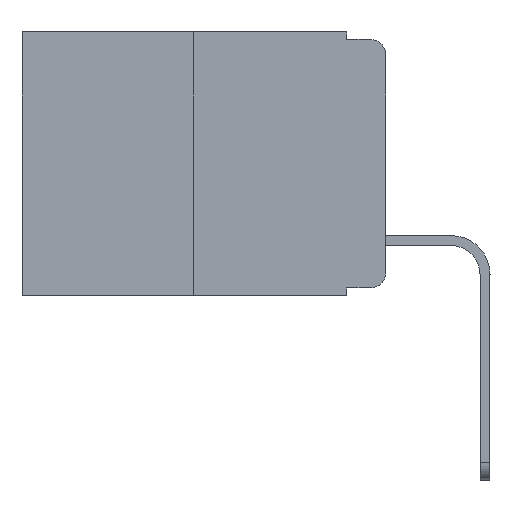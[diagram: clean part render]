
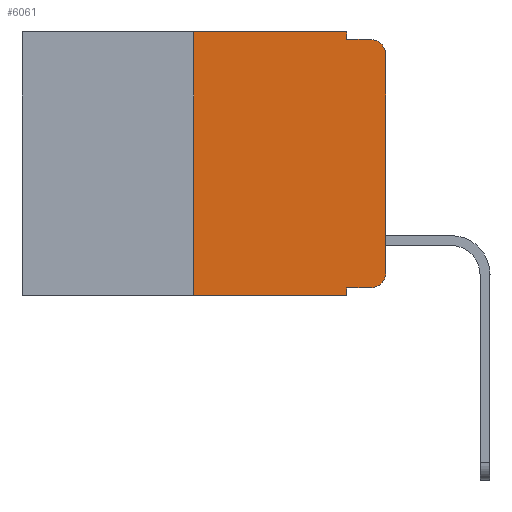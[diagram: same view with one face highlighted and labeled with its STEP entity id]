
A CAD part, left-side view. The second image highlights one B-rep face of the part: STEP entity #6061.
In plain terms, the highlighted planar face has unit normal (-1, 0, 0).
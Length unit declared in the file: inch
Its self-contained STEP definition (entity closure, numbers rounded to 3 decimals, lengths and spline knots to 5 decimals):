
#34 = VECTOR ( 'NONE', #3097, 39.37008 ) ;
#148 = CIRCLE ( 'NONE', #10623, 0.02 ) ;
#178 = ORIENTED_EDGE ( 'NONE', *, *, #2324, .T. ) ;
#459 = LINE ( 'NONE', #8525, #11110 ) ;
#597 = VERTEX_POINT ( 'NONE', #6587 ) ;
#667 = VERTEX_POINT ( 'NONE', #7694 ) ;
#918 = LINE ( 'NONE', #9375, #13182 ) ;
#1344 = EDGE_LOOP ( 'NONE', ( #1775, #178, #8103, #5149, #6812, #6428, #12021, #8382, #8187, #9135 ) ) ;
#1541 = CARTESIAN_POINT ( 'NONE',  ( 0., 0.02, -0.01 ) ) ;
#1775 = ORIENTED_EDGE ( 'NONE', *, *, #5289, .T. ) ;
#2139 = EDGE_CURVE ( 'NONE', #5920, #12277, #10236, .T. ) ;
#2301 = EDGE_CURVE ( 'NONE', #7351, #10772, #459, .T. ) ;
#2324 = EDGE_CURVE ( 'NONE', #7020, #2743, #148, .T. ) ;
#2660 = EDGE_CURVE ( 'NONE', #4343, #11978, #9646, .T. ) ;
#2743 = VERTEX_POINT ( 'NONE', #1541 ) ;
#2759 = CARTESIAN_POINT ( 'NONE',  ( 0., 0.473, 0. ) ) ;
#2847 = VECTOR ( 'NONE', #8816, 39.37008 ) ;
#2946 = DIRECTION ( 'NONE',  ( -1., 0., 0. ) ) ;
#2991 = CIRCLE ( 'NONE', #12866, 0.02 ) ;
#3029 = DIRECTION ( 'NONE',  ( 0., 0., -1. ) ) ;
#3097 = DIRECTION ( 'NONE',  ( 0., -1., 0. ) ) ;
#3358 = VECTOR ( 'NONE', #10687, 39.37008 ) ;
#3482 = LINE ( 'NONE', #8141, #8485 ) ;
#3493 = CARTESIAN_POINT ( 'NONE',  ( 0., 0.051, -0.333 ) ) ;
#3689 = LINE ( 'NONE', #3493, #3358 ) ;
#3695 = VECTOR ( 'NONE', #4351, 39.37008 ) ;
#3797 = DIRECTION ( 'NONE',  ( 0., 0., -1. ) ) ;
#4082 = CARTESIAN_POINT ( 'NONE',  ( 0., 0.051, -0.01 ) ) ;
#4132 = EDGE_CURVE ( 'NONE', #11978, #5920, #918, .T. ) ;
#4182 = CARTESIAN_POINT ( 'NONE',  ( 0., 0.051, -0.333 ) ) ;
#4343 = VERTEX_POINT ( 'NONE', #8898 ) ;
#4351 = DIRECTION ( 'NONE',  ( 0., 0., 1. ) ) ;
#4927 = DIRECTION ( 'NONE',  ( 0., 0., -1. ) ) ;
#5132 = CARTESIAN_POINT ( 'NONE',  ( 0., 0.25, 0. ) ) ;
#5149 = ORIENTED_EDGE ( 'NONE', *, *, #2139, .F. ) ;
#5204 = CARTESIAN_POINT ( 'NONE',  ( 0., 0.051, 0. ) ) ;
#5289 = EDGE_CURVE ( 'NONE', #667, #7020, #3482, .T. ) ;
#5399 = CARTESIAN_POINT ( 'NONE',  ( 0., 0.051, -0.01 ) ) ;
#5708 = FACE_OUTER_BOUND ( 'NONE', #1344, .T. ) ;
#5860 = CARTESIAN_POINT ( 'NONE',  ( 0., 0.25, 0. ) ) ;
#5920 = VERTEX_POINT ( 'NONE', #6330 ) ;
#6061 = ADVANCED_FACE ( 'NONE', ( #5708 ), #6921, .F. ) ;
#6109 = CARTESIAN_POINT ( 'NONE',  ( 0., 0.051, -0.343 ) ) ;
#6330 = CARTESIAN_POINT ( 'NONE',  ( 0., 0.051, 0. ) ) ;
#6428 = ORIENTED_EDGE ( 'NONE', *, *, #2660, .F. ) ;
#6587 = CARTESIAN_POINT ( 'NONE',  ( 0., 0.02, -0.333 ) ) ;
#6812 = ORIENTED_EDGE ( 'NONE', *, *, #4132, .F. ) ;
#6857 = EDGE_CURVE ( 'NONE', #12277, #2743, #13115, .T. ) ;
#6921 = PLANE ( 'NONE',  #10375 ) ;
#7020 = VERTEX_POINT ( 'NONE', #7466 ) ;
#7351 = VERTEX_POINT ( 'NONE', #4182 ) ;
#7466 = CARTESIAN_POINT ( 'NONE',  ( 0., 0., -0.03 ) ) ;
#7655 = CARTESIAN_POINT ( 'NONE',  ( 0., 0.473, -0.343 ) ) ;
#7694 = CARTESIAN_POINT ( 'NONE',  ( 0., 0., -0.313 ) ) ;
#8103 = ORIENTED_EDGE ( 'NONE', *, *, #6857, .F. ) ;
#8141 = CARTESIAN_POINT ( 'NONE',  ( 0., 0., 0. ) ) ;
#8187 = ORIENTED_EDGE ( 'NONE', *, *, #11074, .T. ) ;
#8332 = LINE ( 'NONE', #7655, #2847 ) ;
#8382 = ORIENTED_EDGE ( 'NONE', *, *, #2301, .F. ) ;
#8400 = DIRECTION ( 'NONE',  ( -1., 0., 0. ) ) ;
#8485 = VECTOR ( 'NONE', #11228, 39.37008 ) ;
#8525 = CARTESIAN_POINT ( 'NONE',  ( 0., 0.051, 0. ) ) ;
#8816 = DIRECTION ( 'NONE',  ( 0., -1., 0. ) ) ;
#8898 = CARTESIAN_POINT ( 'NONE',  ( 0., 0.25, -0.343 ) ) ;
#9135 = ORIENTED_EDGE ( 'NONE', *, *, #13073, .T. ) ;
#9375 = CARTESIAN_POINT ( 'NONE',  ( 0., 0.473, 0. ) ) ;
#9524 = DIRECTION ( 'NONE',  ( 0., -1., 0. ) ) ;
#9646 = LINE ( 'NONE', #5132, #3695 ) ;
#10236 = LINE ( 'NONE', #5204, #11054 ) ;
#10375 = AXIS2_PLACEMENT_3D ( 'NONE', #2759, #13169, #3797 ) ;
#10496 = CARTESIAN_POINT ( 'NONE',  ( 0., 0.02, -0.03 ) ) ;
#10623 = AXIS2_PLACEMENT_3D ( 'NONE', #10496, #8400, #11628 ) ;
#10687 = DIRECTION ( 'NONE',  ( 0., -1., 0. ) ) ;
#10772 = VERTEX_POINT ( 'NONE', #6109 ) ;
#11054 = VECTOR ( 'NONE', #3029, 39.37008 ) ;
#11074 = EDGE_CURVE ( 'NONE', #7351, #597, #3689, .T. ) ;
#11110 = VECTOR ( 'NONE', #12495, 39.37008 ) ;
#11228 = DIRECTION ( 'NONE',  ( 0., 0., 1. ) ) ;
#11628 = DIRECTION ( 'NONE',  ( 0., 0., -1. ) ) ;
#11978 = VERTEX_POINT ( 'NONE', #5860 ) ;
#12021 = ORIENTED_EDGE ( 'NONE', *, *, #12347, .T. ) ;
#12105 = CARTESIAN_POINT ( 'NONE',  ( 0., 0.02, -0.313 ) ) ;
#12277 = VERTEX_POINT ( 'NONE', #5399 ) ;
#12347 = EDGE_CURVE ( 'NONE', #4343, #10772, #8332, .T. ) ;
#12495 = DIRECTION ( 'NONE',  ( 0., 0., -1. ) ) ;
#12866 = AXIS2_PLACEMENT_3D ( 'NONE', #12105, #2946, #4927 ) ;
#13073 = EDGE_CURVE ( 'NONE', #597, #667, #2991, .T. ) ;
#13115 = LINE ( 'NONE', #4082, #34 ) ;
#13169 = DIRECTION ( 'NONE',  ( 1., 0., 0. ) ) ;
#13182 = VECTOR ( 'NONE', #9524, 39.37008 ) ;
